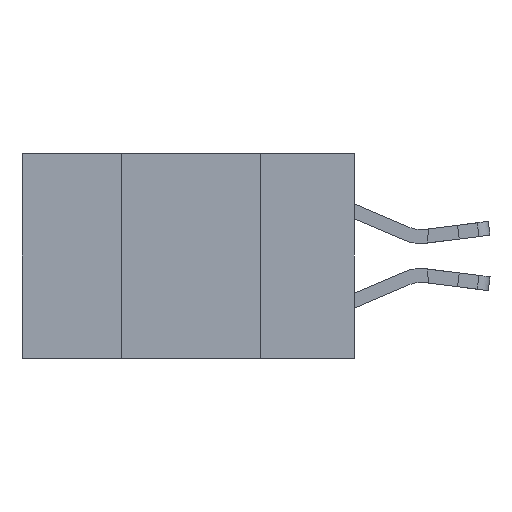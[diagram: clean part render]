
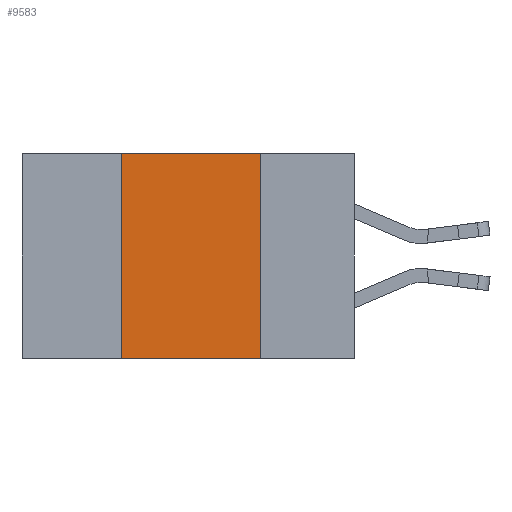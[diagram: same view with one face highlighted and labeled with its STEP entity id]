
A CAD part, left-side view. The second image highlights one B-rep face of the part: STEP entity #9583.
In plain terms, the highlighted planar face has unit normal (-1, 0, 0).
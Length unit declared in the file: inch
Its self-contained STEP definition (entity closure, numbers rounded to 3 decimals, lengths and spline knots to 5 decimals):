
#13 = DIRECTION ( 'NONE',  ( 0., 0., -1. ) ) ;
#105 = EDGE_LOOP ( 'NONE', ( #12493, #7608, #11918, #3300 ) ) ;
#128 = VECTOR ( 'NONE', #13, 39.37008 ) ;
#963 = DIRECTION ( 'NONE',  ( 1., 0., 0. ) ) ;
#1002 = PLANE ( 'NONE',  #12539 ) ;
#1820 = VERTEX_POINT ( 'NONE', #6304 ) ;
#2356 = DIRECTION ( 'NONE',  ( 0., -1., 0. ) ) ;
#2516 = EDGE_CURVE ( 'NONE', #1820, #11007, #2932, .T. ) ;
#2668 = FACE_OUTER_BOUND ( 'NONE', #105, .T. ) ;
#2714 = VERTEX_POINT ( 'NONE', #13063 ) ;
#2932 = LINE ( 'NONE', #11455, #128 ) ;
#3032 = CARTESIAN_POINT ( 'NONE',  ( 0., 0.6, 0. ) ) ;
#3300 = ORIENTED_EDGE ( 'NONE', *, *, #11315, .T. ) ;
#3607 = CARTESIAN_POINT ( 'NONE',  ( 0., 0.6, 0. ) ) ;
#4437 = EDGE_CURVE ( 'NONE', #11513, #1820, #10813, .T. ) ;
#4991 = CARTESIAN_POINT ( 'NONE',  ( 0., 0.42, 0. ) ) ;
#5401 = CARTESIAN_POINT ( 'NONE',  ( 0., 0.42, 0. ) ) ;
#6280 = CARTESIAN_POINT ( 'NONE',  ( 0., 0.17, -0.37 ) ) ;
#6304 = CARTESIAN_POINT ( 'NONE',  ( 0., 0.17, 0. ) ) ;
#6430 = VECTOR ( 'NONE', #7417, 39.37008 ) ;
#7417 = DIRECTION ( 'NONE',  ( 0., 0., 1. ) ) ;
#7608 = ORIENTED_EDGE ( 'NONE', *, *, #4437, .F. ) ;
#7653 = EDGE_CURVE ( 'NONE', #2714, #11513, #13345, .T. ) ;
#9583 = ADVANCED_FACE ( 'NONE', ( #2668 ), #1002, .F. ) ;
#10192 = LINE ( 'NONE', #12812, #12304 ) ;
#10444 = DIRECTION ( 'NONE',  ( 0., 0., -1. ) ) ;
#10813 = LINE ( 'NONE', #3607, #11934 ) ;
#11007 = VERTEX_POINT ( 'NONE', #6280 ) ;
#11315 = EDGE_CURVE ( 'NONE', #2714, #11007, #10192, .T. ) ;
#11455 = CARTESIAN_POINT ( 'NONE',  ( 0., 0.17, 0. ) ) ;
#11513 = VERTEX_POINT ( 'NONE', #4991 ) ;
#11918 = ORIENTED_EDGE ( 'NONE', *, *, #7653, .F. ) ;
#11934 = VECTOR ( 'NONE', #12058, 39.37008 ) ;
#12058 = DIRECTION ( 'NONE',  ( 0., -1., 0. ) ) ;
#12304 = VECTOR ( 'NONE', #2356, 39.37008 ) ;
#12493 = ORIENTED_EDGE ( 'NONE', *, *, #2516, .F. ) ;
#12539 = AXIS2_PLACEMENT_3D ( 'NONE', #3032, #963, #10444 ) ;
#12812 = CARTESIAN_POINT ( 'NONE',  ( 0., 0.6, -0.37 ) ) ;
#13063 = CARTESIAN_POINT ( 'NONE',  ( 0., 0.42, -0.37 ) ) ;
#13345 = LINE ( 'NONE', #5401, #6430 ) ;
